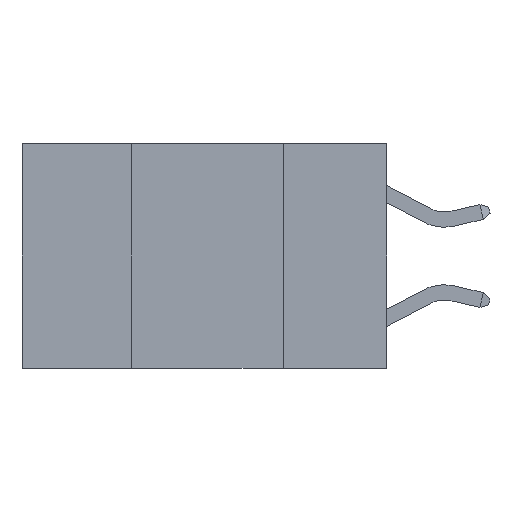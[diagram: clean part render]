
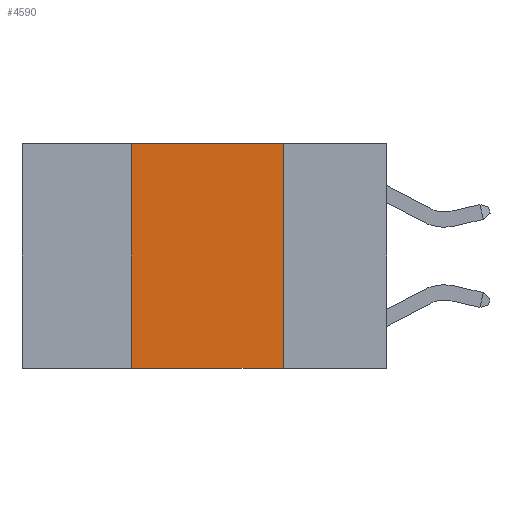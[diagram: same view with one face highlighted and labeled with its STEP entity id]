
A CAD part, left-side view. The second image highlights one B-rep face of the part: STEP entity #4590.
In plain terms, the highlighted planar face has unit normal (-1, 0, 0).
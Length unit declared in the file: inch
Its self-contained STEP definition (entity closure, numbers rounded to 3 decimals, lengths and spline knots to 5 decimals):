
#252 = DIRECTION ( 'NONE',  ( 0., -1., 0. ) ) ;
#763 = CARTESIAN_POINT ( 'NONE',  ( 0., 0.17, 0. ) ) ;
#829 = VECTOR ( 'NONE', #6648, 39.37008 ) ;
#1352 = LINE ( 'NONE', #3926, #829 ) ;
#1642 = DIRECTION ( 'NONE',  ( 1., 0., 0. ) ) ;
#1735 = LINE ( 'NONE', #763, #2412 ) ;
#1879 = CARTESIAN_POINT ( 'NONE',  ( 0., 0.42, 0. ) ) ;
#2020 = VERTEX_POINT ( 'NONE', #8130 ) ;
#2347 = DIRECTION ( 'NONE',  ( 0., 0., -1. ) ) ;
#2399 = EDGE_CURVE ( 'NONE', #4327, #7584, #8418, .T. ) ;
#2412 = VECTOR ( 'NONE', #3554, 39.37008 ) ;
#2453 = PLANE ( 'NONE',  #5664 ) ;
#2822 = CARTESIAN_POINT ( 'NONE',  ( 0., 0.42, 0. ) ) ;
#2912 = ORIENTED_EDGE ( 'NONE', *, *, #5597, .T. ) ;
#3374 = EDGE_CURVE ( 'NONE', #7584, #2020, #1352, .T. ) ;
#3550 = CARTESIAN_POINT ( 'NONE',  ( 0., 0.6, -0.37 ) ) ;
#3554 = DIRECTION ( 'NONE',  ( 0., 0., -1. ) ) ;
#3558 = EDGE_CURVE ( 'NONE', #2020, #6099, #1735, .T. ) ;
#3873 = ORIENTED_EDGE ( 'NONE', *, *, #3558, .F. ) ;
#3926 = CARTESIAN_POINT ( 'NONE',  ( 0., 0.6, 0. ) ) ;
#4322 = LINE ( 'NONE', #3550, #7530 ) ;
#4327 = VERTEX_POINT ( 'NONE', #5940 ) ;
#4553 = CARTESIAN_POINT ( 'NONE',  ( 0., 0.17, -0.37 ) ) ;
#4590 = ADVANCED_FACE ( 'NONE', ( #7295 ), #2453, .F. ) ;
#4780 = ORIENTED_EDGE ( 'NONE', *, *, #2399, .F. ) ;
#5597 = EDGE_CURVE ( 'NONE', #4327, #6099, #4322, .T. ) ;
#5664 = AXIS2_PLACEMENT_3D ( 'NONE', #5711, #1642, #2347 ) ;
#5711 = CARTESIAN_POINT ( 'NONE',  ( 0., 0.6, 0. ) ) ;
#5940 = CARTESIAN_POINT ( 'NONE',  ( 0., 0.42, -0.37 ) ) ;
#6080 = DIRECTION ( 'NONE',  ( 0., 0., 1. ) ) ;
#6099 = VERTEX_POINT ( 'NONE', #4553 ) ;
#6568 = EDGE_LOOP ( 'NONE', ( #3873, #8865, #4780, #2912 ) ) ;
#6648 = DIRECTION ( 'NONE',  ( 0., -1., 0. ) ) ;
#7295 = FACE_OUTER_BOUND ( 'NONE', #6568, .T. ) ;
#7530 = VECTOR ( 'NONE', #252, 39.37008 ) ;
#7584 = VERTEX_POINT ( 'NONE', #1879 ) ;
#8130 = CARTESIAN_POINT ( 'NONE',  ( 0., 0.17, 0. ) ) ;
#8418 = LINE ( 'NONE', #2822, #9397 ) ;
#8865 = ORIENTED_EDGE ( 'NONE', *, *, #3374, .F. ) ;
#9397 = VECTOR ( 'NONE', #6080, 39.37008 ) ;
